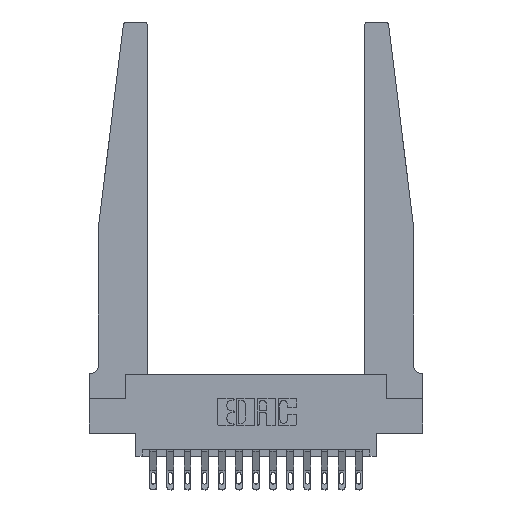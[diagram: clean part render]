
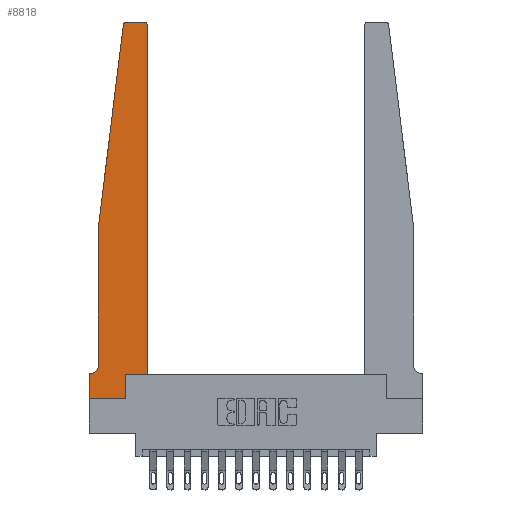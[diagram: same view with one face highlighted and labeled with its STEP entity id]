
A CAD part, top view. The second image highlights one B-rep face of the part: STEP entity #8818.
In plain terms, the highlighted planar face has unit normal (0, 0, 1).
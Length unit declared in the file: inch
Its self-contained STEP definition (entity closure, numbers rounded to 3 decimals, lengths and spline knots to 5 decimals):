
#34 = ORIENTED_EDGE ( 'NONE', *, *, #11451, .T. ) ;
#878 = VERTEX_POINT ( 'NONE', #15236 ) ;
#1000 = VECTOR ( 'NONE', #9350, 39.37008 ) ;
#1161 = CARTESIAN_POINT ( 'NONE',  ( 0.395, 2.75, 0.37 ) ) ;
#1607 = ORIENTED_EDGE ( 'NONE', *, *, #5702, .T. ) ;
#1676 = LINE ( 'NONE', #17033, #8103 ) ;
#2087 = VERTEX_POINT ( 'NONE', #3484 ) ;
#2302 = ORIENTED_EDGE ( 'NONE', *, *, #13702, .T. ) ;
#2545 = CARTESIAN_POINT ( 'NONE',  ( 0.425, 0.18, 0.37 ) ) ;
#2823 = ORIENTED_EDGE ( 'NONE', *, *, #12298, .T. ) ;
#3084 = LINE ( 'NONE', #7188, #3995 ) ;
#3100 = VECTOR ( 'NONE', #16067, 39.37008 ) ;
#3465 = DIRECTION ( 'NONE',  ( 1., 0., 0. ) ) ;
#3484 = CARTESIAN_POINT ( 'NONE',  ( 0., 0., 0.37 ) ) ;
#3502 = EDGE_CURVE ( 'NONE', #4593, #4989, #1676, .T. ) ;
#3725 = AXIS2_PLACEMENT_3D ( 'NONE', #8718, #12752, #15695 ) ;
#3995 = VECTOR ( 'NONE', #4284, 39.37008 ) ;
#4097 = VECTOR ( 'NONE', #3465, 39.37008 ) ;
#4187 = CARTESIAN_POINT ( 'NONE',  ( 0.015, 0.1875, 0.37 ) ) ;
#4284 = DIRECTION ( 'NONE',  ( 1., 0., 0. ) ) ;
#4367 = VERTEX_POINT ( 'NONE', #5244 ) ;
#4593 = VERTEX_POINT ( 'NONE', #13551 ) ;
#4898 = CIRCLE ( 'NONE', #3725, 0.05 ) ;
#4989 = VERTEX_POINT ( 'NONE', #11882 ) ;
#5146 = VECTOR ( 'NONE', #11049, 39.37008 ) ;
#5244 = CARTESIAN_POINT ( 'NONE',  ( 0.2605, 0.18, 0.37 ) ) ;
#5314 = ORIENTED_EDGE ( 'NONE', *, *, #14334, .T. ) ;
#5702 = EDGE_CURVE ( 'NONE', #14782, #9429, #17487, .T. ) ;
#5799 = DIRECTION ( 'NONE',  ( 0., 0., 1. ) ) ;
#6204 = VERTEX_POINT ( 'NONE', #4187 ) ;
#6234 = VERTEX_POINT ( 'NONE', #16808 ) ;
#6744 = ORIENTED_EDGE ( 'NONE', *, *, #9581, .T. ) ;
#6770 = EDGE_CURVE ( 'NONE', #4989, #6204, #4898, .T. ) ;
#7097 = ORIENTED_EDGE ( 'NONE', *, *, #11332, .T. ) ;
#7175 = LINE ( 'NONE', #8561, #8651 ) ;
#7188 = CARTESIAN_POINT ( 'NONE',  ( 0.425, 0.18, 0.37 ) ) ;
#7744 = LINE ( 'NONE', #13079, #4097 ) ;
#8081 = CIRCLE ( 'NONE', #8380, 0.03 ) ;
#8103 = VECTOR ( 'NONE', #11457, 39.37008 ) ;
#8106 = CARTESIAN_POINT ( 'NONE',  ( 0.2605, 0.18, 0.37 ) ) ;
#8132 = DIRECTION ( 'NONE',  ( 1., 0., 0. ) ) ;
#8371 = DIRECTION ( 'NONE',  ( 0., -1., 0. ) ) ;
#8380 = AXIS2_PLACEMENT_3D ( 'NONE', #13063, #14633, #17358 ) ;
#8561 = CARTESIAN_POINT ( 'NONE',  ( 0., 0., 0.37 ) ) ;
#8651 = VECTOR ( 'NONE', #8371, 39.37008 ) ;
#8718 = CARTESIAN_POINT ( 'NONE',  ( 0.015, 0.2375, 0.37 ) ) ;
#8793 = ORIENTED_EDGE ( 'NONE', *, *, #12527, .T. ) ;
#8818 = ADVANCED_FACE ( 'NONE', ( #10530 ), #12363, .T. ) ;
#8854 = ORIENTED_EDGE ( 'NONE', *, *, #6770, .T. ) ;
#9289 = VECTOR ( 'NONE', #17304, 39.37008 ) ;
#9350 = DIRECTION ( 'NONE',  ( -1., 0., 0. ) ) ;
#9429 = VERTEX_POINT ( 'NONE', #10080 ) ;
#9581 = EDGE_CURVE ( 'NONE', #2087, #878, #7744, .T. ) ;
#9707 = CARTESIAN_POINT ( 'NONE',  ( 0., 0.1875, 0.37 ) ) ;
#10080 = CARTESIAN_POINT ( 'NONE',  ( 0.27653, 2.75, 0.37 ) ) ;
#10159 = AXIS2_PLACEMENT_3D ( 'NONE', #15461, #5799, #16999 ) ;
#10223 = CARTESIAN_POINT ( 'NONE',  ( 0.24675, 2.72367, 0.37 ) ) ;
#10530 = FACE_OUTER_BOUND ( 'NONE', #10771, .T. ) ;
#10771 = EDGE_LOOP ( 'NONE', ( #1607, #2823, #16767, #17803, #8854, #2302, #34, #6744, #7097, #5314, #8793, #14560 ) ) ;
#11049 = DIRECTION ( 'NONE',  ( 0., 1., 0. ) ) ;
#11332 = EDGE_CURVE ( 'NONE', #878, #4367, #12138, .T. ) ;
#11363 = AXIS2_PLACEMENT_3D ( 'NONE', #9707, #13912, #8132 ) ;
#11451 = EDGE_CURVE ( 'NONE', #6234, #2087, #7175, .T. ) ;
#11457 = DIRECTION ( 'NONE',  ( 0., -1., 0. ) ) ;
#11528 = EDGE_CURVE ( 'NONE', #12699, #4593, #17335, .T. ) ;
#11587 = CARTESIAN_POINT ( 'NONE',  ( 0.065, 1.25, 0.37 ) ) ;
#11882 = CARTESIAN_POINT ( 'NONE',  ( 0.065, 0.2375, 0.37 ) ) ;
#11883 = CIRCLE ( 'NONE', #10159, 0.03 ) ;
#12057 = CARTESIAN_POINT ( 'NONE',  ( 0.425, 0.18, 0.37 ) ) ;
#12138 = LINE ( 'NONE', #8106, #13027 ) ;
#12298 = EDGE_CURVE ( 'NONE', #9429, #12699, #8081, .T. ) ;
#12363 = PLANE ( 'NONE',  #11363 ) ;
#12431 = VERTEX_POINT ( 'NONE', #12057 ) ;
#12445 = VERTEX_POINT ( 'NONE', #15086 ) ;
#12527 = EDGE_CURVE ( 'NONE', #12431, #12445, #16464, .T. ) ;
#12648 = EDGE_CURVE ( 'NONE', #12445, #14782, #11883, .T. ) ;
#12699 = VERTEX_POINT ( 'NONE', #10223 ) ;
#12752 = DIRECTION ( 'NONE',  ( 0., 0., -1. ) ) ;
#13027 = VECTOR ( 'NONE', #17893, 39.37008 ) ;
#13063 = CARTESIAN_POINT ( 'NONE',  ( 0.27653, 2.72, 0.37 ) ) ;
#13079 = CARTESIAN_POINT ( 'NONE',  ( 0., 0., 0.37 ) ) ;
#13551 = CARTESIAN_POINT ( 'NONE',  ( 0.065, 1.25, 0.37 ) ) ;
#13702 = EDGE_CURVE ( 'NONE', #6204, #6234, #14661, .T. ) ;
#13912 = DIRECTION ( 'NONE',  ( 0., 0., 1. ) ) ;
#14334 = EDGE_CURVE ( 'NONE', #4367, #12431, #3084, .T. ) ;
#14560 = ORIENTED_EDGE ( 'NONE', *, *, #12648, .T. ) ;
#14633 = DIRECTION ( 'NONE',  ( 0., 0., 1. ) ) ;
#14661 = LINE ( 'NONE', #15858, #9289 ) ;
#14782 = VERTEX_POINT ( 'NONE', #1161 ) ;
#15086 = CARTESIAN_POINT ( 'NONE',  ( 0.425, 2.72, 0.37 ) ) ;
#15236 = CARTESIAN_POINT ( 'NONE',  ( 0.2605, 0., 0.37 ) ) ;
#15461 = CARTESIAN_POINT ( 'NONE',  ( 0.395, 2.72, 0.37 ) ) ;
#15695 = DIRECTION ( 'NONE',  ( -1., 0., 0. ) ) ;
#15858 = CARTESIAN_POINT ( 'NONE',  ( 0.065, 0.1875, 0.37 ) ) ;
#16067 = DIRECTION ( 'NONE',  ( -0.122, -0.992, 0. ) ) ;
#16464 = LINE ( 'NONE', #2545, #5146 ) ;
#16767 = ORIENTED_EDGE ( 'NONE', *, *, #11528, .T. ) ;
#16808 = CARTESIAN_POINT ( 'NONE',  ( 0., 0.1875, 0.37 ) ) ;
#16999 = DIRECTION ( 'NONE',  ( 1., 0., 0. ) ) ;
#17033 = CARTESIAN_POINT ( 'NONE',  ( 0.065, 1.25, 0.37 ) ) ;
#17304 = DIRECTION ( 'NONE',  ( -1., 0., 0. ) ) ;
#17335 = LINE ( 'NONE', #11587, #3100 ) ;
#17358 = DIRECTION ( 'NONE',  ( 1., 0., 0. ) ) ;
#17487 = LINE ( 'NONE', #17759, #1000 ) ;
#17759 = CARTESIAN_POINT ( 'NONE',  ( 0.25, 2.75, 0.37 ) ) ;
#17803 = ORIENTED_EDGE ( 'NONE', *, *, #3502, .T. ) ;
#17893 = DIRECTION ( 'NONE',  ( 0., 1., 0. ) ) ;
